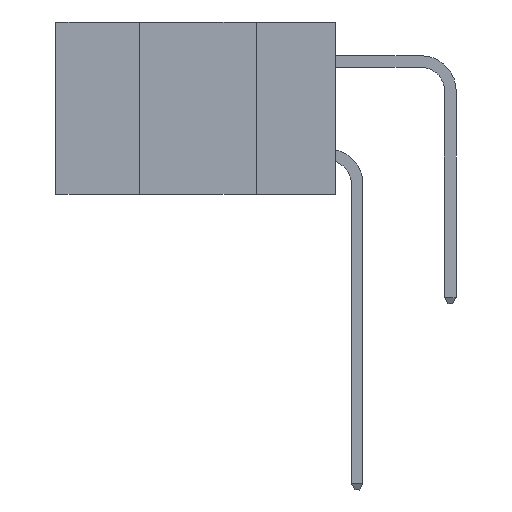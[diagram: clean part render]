
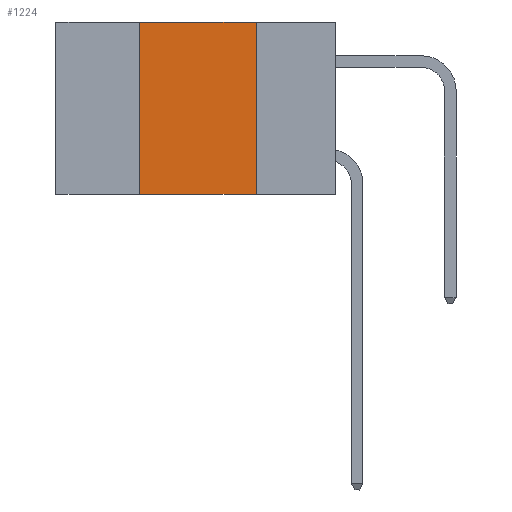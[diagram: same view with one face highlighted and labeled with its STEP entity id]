
A CAD part, left-side view. The second image highlights one B-rep face of the part: STEP entity #1224.
In plain terms, the highlighted planar face has unit normal (-1, 0, 0).
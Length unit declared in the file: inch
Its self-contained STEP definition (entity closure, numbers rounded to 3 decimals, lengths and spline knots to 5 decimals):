
#332 = CARTESIAN_POINT ( 'NONE',  ( 0., 0.42, 0. ) ) ;
#816 = DIRECTION ( 'NONE',  ( 0., 0., -1. ) ) ;
#1049 = CARTESIAN_POINT ( 'NONE',  ( 0., 0.42, 0. ) ) ;
#1055 = EDGE_LOOP ( 'NONE', ( #10250, #4903, #8435, #7923 ) ) ;
#1224 = ADVANCED_FACE ( 'NONE', ( #10706 ), #5590, .F. ) ;
#1650 = LINE ( 'NONE', #2387, #8196 ) ;
#1834 = DIRECTION ( 'NONE',  ( 0., 0., 1. ) ) ;
#2024 = CARTESIAN_POINT ( 'NONE',  ( 0., 0.6, 0. ) ) ;
#2387 = CARTESIAN_POINT ( 'NONE',  ( 0., 0.17, 0. ) ) ;
#2684 = LINE ( 'NONE', #1049, #7447 ) ;
#3048 = CARTESIAN_POINT ( 'NONE',  ( 0., 0.6, 0. ) ) ;
#3226 = CARTESIAN_POINT ( 'NONE',  ( 0., 0.17, 0. ) ) ;
#3793 = DIRECTION ( 'NONE',  ( 0., 0., -1. ) ) ;
#3832 = LINE ( 'NONE', #2024, #9475 ) ;
#4091 = CARTESIAN_POINT ( 'NONE',  ( 0., 0.17, -0.37 ) ) ;
#4742 = DIRECTION ( 'NONE',  ( 1., 0., 0. ) ) ;
#4875 = EDGE_CURVE ( 'NONE', #9344, #10405, #2684, .T. ) ;
#4903 = ORIENTED_EDGE ( 'NONE', *, *, #9836, .F. ) ;
#5428 = VERTEX_POINT ( 'NONE', #4091 ) ;
#5455 = DIRECTION ( 'NONE',  ( 0., -1., 0. ) ) ;
#5590 = PLANE ( 'NONE',  #5631 ) ;
#5631 = AXIS2_PLACEMENT_3D ( 'NONE', #3048, #4742, #3793 ) ;
#5633 = EDGE_CURVE ( 'NONE', #9344, #5428, #6046, .T. ) ;
#6046 = LINE ( 'NONE', #7838, #8183 ) ;
#6671 = CARTESIAN_POINT ( 'NONE',  ( 0., 0.42, -0.37 ) ) ;
#7045 = DIRECTION ( 'NONE',  ( 0., -1., 0. ) ) ;
#7182 = VERTEX_POINT ( 'NONE', #3226 ) ;
#7447 = VECTOR ( 'NONE', #1834, 39.37008 ) ;
#7838 = CARTESIAN_POINT ( 'NONE',  ( 0., 0.6, -0.37 ) ) ;
#7923 = ORIENTED_EDGE ( 'NONE', *, *, #5633, .T. ) ;
#8183 = VECTOR ( 'NONE', #7045, 39.37008 ) ;
#8196 = VECTOR ( 'NONE', #816, 39.37008 ) ;
#8435 = ORIENTED_EDGE ( 'NONE', *, *, #4875, .F. ) ;
#9344 = VERTEX_POINT ( 'NONE', #6671 ) ;
#9475 = VECTOR ( 'NONE', #5455, 39.37008 ) ;
#9716 = EDGE_CURVE ( 'NONE', #7182, #5428, #1650, .T. ) ;
#9836 = EDGE_CURVE ( 'NONE', #10405, #7182, #3832, .T. ) ;
#10250 = ORIENTED_EDGE ( 'NONE', *, *, #9716, .F. ) ;
#10405 = VERTEX_POINT ( 'NONE', #332 ) ;
#10706 = FACE_OUTER_BOUND ( 'NONE', #1055, .T. ) ;
